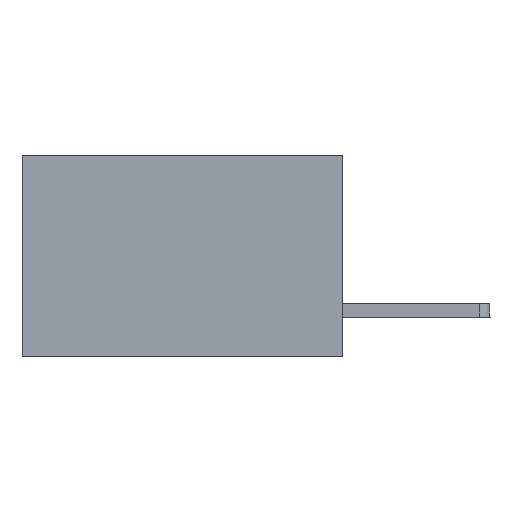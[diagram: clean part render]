
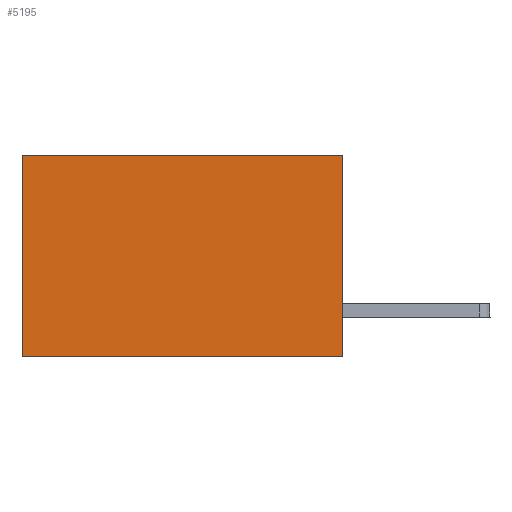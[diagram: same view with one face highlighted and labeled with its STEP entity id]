
A CAD part, left-side view. The second image highlights one B-rep face of the part: STEP entity #5195.
In plain terms, the highlighted planar face has unit normal (-1, 0, 0).
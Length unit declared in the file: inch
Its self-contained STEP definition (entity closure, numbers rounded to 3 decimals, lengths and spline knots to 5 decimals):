
#693 = ORIENTED_EDGE ( 'NONE', *, *, #1438, .F. ) ;
#736 = ORIENTED_EDGE ( 'NONE', *, *, #3246, .T. ) ;
#1121 = DIRECTION ( 'NONE',  ( 1., 0., 0. ) ) ;
#1312 = VERTEX_POINT ( 'NONE', #2708 ) ;
#1405 = DIRECTION ( 'NONE',  ( 0., 0., -1. ) ) ;
#1438 = EDGE_CURVE ( 'NONE', #1312, #11003, #9305, .T. ) ;
#1469 = CARTESIAN_POINT ( 'NONE',  ( 0.277, 0.59, -0.37 ) ) ;
#2137 = CARTESIAN_POINT ( 'NONE',  ( 0.277, 0.59, 0. ) ) ;
#2198 = DIRECTION ( 'NONE',  ( 0., 0., -1. ) ) ;
#2460 = ORIENTED_EDGE ( 'NONE', *, *, #5460, .F. ) ;
#2468 = EDGE_LOOP ( 'NONE', ( #3568, #2460, #693, #736 ) ) ;
#2708 = CARTESIAN_POINT ( 'NONE',  ( 0.277, 0., 0. ) ) ;
#3246 = EDGE_CURVE ( 'NONE', #1312, #9506, #7689, .T. ) ;
#3564 = VERTEX_POINT ( 'NONE', #5995 ) ;
#3568 = ORIENTED_EDGE ( 'NONE', *, *, #5416, .T. ) ;
#4125 = AXIS2_PLACEMENT_3D ( 'NONE', #8229, #1121, #5500 ) ;
#4308 = VECTOR ( 'NONE', #1405, 39.37008 ) ;
#5195 = ADVANCED_FACE ( 'NONE', ( #10068 ), #6565, .F. ) ;
#5416 = EDGE_CURVE ( 'NONE', #9506, #3564, #10481, .T. ) ;
#5437 = VECTOR ( 'NONE', #11313, 39.37008 ) ;
#5460 = EDGE_CURVE ( 'NONE', #11003, #3564, #7748, .T. ) ;
#5500 = DIRECTION ( 'NONE',  ( 0., 0., -1. ) ) ;
#5995 = CARTESIAN_POINT ( 'NONE',  ( 0.277, 0.59, -0.37 ) ) ;
#6565 = PLANE ( 'NONE',  #4125 ) ;
#6853 = CARTESIAN_POINT ( 'NONE',  ( 0.277, 0., -0.37 ) ) ;
#7689 = LINE ( 'NONE', #11312, #10321 ) ;
#7748 = LINE ( 'NONE', #6853, #5437 ) ;
#8229 = CARTESIAN_POINT ( 'NONE',  ( 0.277, 0., -0.37 ) ) ;
#8345 = CARTESIAN_POINT ( 'NONE',  ( 0.277, 0., -0.37 ) ) ;
#9305 = LINE ( 'NONE', #8345, #10303 ) ;
#9474 = DIRECTION ( 'NONE',  ( 0., 1., 0. ) ) ;
#9506 = VERTEX_POINT ( 'NONE', #2137 ) ;
#10068 = FACE_OUTER_BOUND ( 'NONE', #2468, .T. ) ;
#10303 = VECTOR ( 'NONE', #2198, 39.37008 ) ;
#10321 = VECTOR ( 'NONE', #9474, 39.37008 ) ;
#10481 = LINE ( 'NONE', #1469, #4308 ) ;
#11003 = VERTEX_POINT ( 'NONE', #11533 ) ;
#11312 = CARTESIAN_POINT ( 'NONE',  ( 0.277, 0., 0. ) ) ;
#11313 = DIRECTION ( 'NONE',  ( 0., 1., 0. ) ) ;
#11533 = CARTESIAN_POINT ( 'NONE',  ( 0.277, 0., -0.37 ) ) ;
